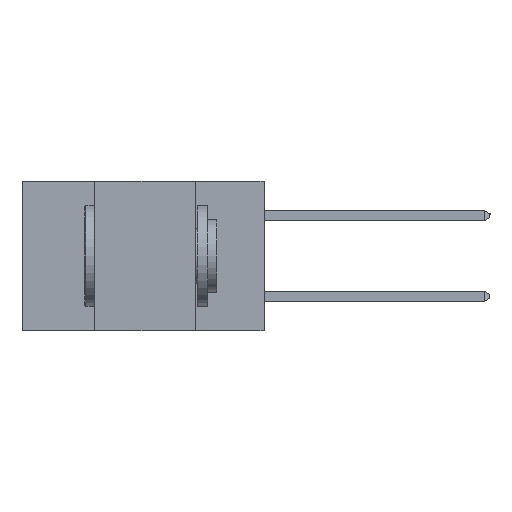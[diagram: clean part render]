
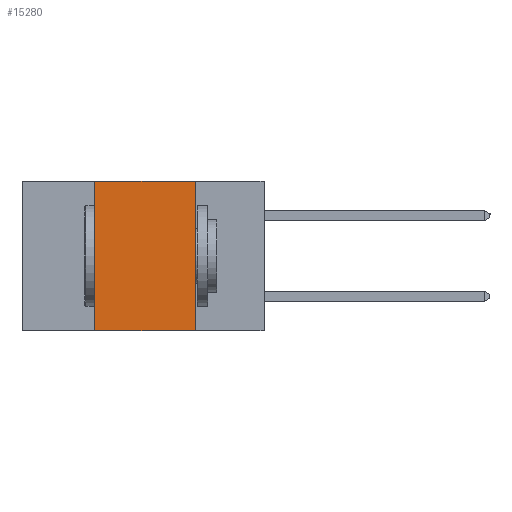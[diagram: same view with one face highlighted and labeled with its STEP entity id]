
A CAD part, left-side view. The second image highlights one B-rep face of the part: STEP entity #15280.
In plain terms, the highlighted planar face has unit normal (-1, 0, 0).
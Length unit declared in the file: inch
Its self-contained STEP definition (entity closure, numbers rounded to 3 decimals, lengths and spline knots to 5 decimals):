
#152 = VECTOR ( 'NONE', #7251, 39.37008 ) ;
#1345 = CARTESIAN_POINT ( 'NONE',  ( 0., 0.17, -0.37 ) ) ;
#1378 = LINE ( 'NONE', #11375, #9827 ) ;
#1451 = DIRECTION ( 'NONE',  ( 0., 0., -1. ) ) ;
#1752 = CARTESIAN_POINT ( 'NONE',  ( 0., 0.17, -0.37 ) ) ;
#1892 = VERTEX_POINT ( 'NONE', #1752 ) ;
#3123 = CARTESIAN_POINT ( 'NONE',  ( 0., 0.42, -0.37 ) ) ;
#3785 = CARTESIAN_POINT ( 'NONE',  ( 0., 0.6, 0. ) ) ;
#4193 = ORIENTED_EDGE ( 'NONE', *, *, #11091, .T. ) ;
#4452 = EDGE_CURVE ( 'NONE', #10727, #8131, #10436, .T. ) ;
#5582 = EDGE_CURVE ( 'NONE', #8131, #6044, #1378, .T. ) ;
#5642 = PLANE ( 'NONE',  #15953 ) ;
#6044 = VERTEX_POINT ( 'NONE', #7387 ) ;
#6091 = CARTESIAN_POINT ( 'NONE',  ( 0., 0.42, -0.37 ) ) ;
#6662 = ORIENTED_EDGE ( 'NONE', *, *, #5582, .F. ) ;
#6948 = DIRECTION ( 'NONE',  ( 0., 0., -1. ) ) ;
#7251 = DIRECTION ( 'NONE',  ( 0., 0., 1. ) ) ;
#7276 = FACE_OUTER_BOUND ( 'NONE', #17084, .T. ) ;
#7387 = CARTESIAN_POINT ( 'NONE',  ( 0., 0.17, 0. ) ) ;
#7412 = LINE ( 'NONE', #1345, #16941 ) ;
#8131 = VERTEX_POINT ( 'NONE', #14866 ) ;
#9384 = DIRECTION ( 'NONE',  ( 0., -1., 0. ) ) ;
#9674 = CARTESIAN_POINT ( 'NONE',  ( 0., 0.6, -0.37 ) ) ;
#9827 = VECTOR ( 'NONE', #9384, 39.37008 ) ;
#10436 = LINE ( 'NONE', #3123, #152 ) ;
#10727 = VERTEX_POINT ( 'NONE', #6091 ) ;
#10775 = ORIENTED_EDGE ( 'NONE', *, *, #13693, .F. ) ;
#11091 = EDGE_CURVE ( 'NONE', #10727, #1892, #13122, .T. ) ;
#11375 = CARTESIAN_POINT ( 'NONE',  ( 0., 0.6, 0. ) ) ;
#12312 = VECTOR ( 'NONE', #16419, 39.37008 ) ;
#13122 = LINE ( 'NONE', #9674, #12312 ) ;
#13693 = EDGE_CURVE ( 'NONE', #6044, #1892, #7412, .T. ) ;
#14866 = CARTESIAN_POINT ( 'NONE',  ( 0., 0.42, 0. ) ) ;
#15280 = ADVANCED_FACE ( 'NONE', ( #7276 ), #5642, .F. ) ;
#15733 = ORIENTED_EDGE ( 'NONE', *, *, #4452, .F. ) ;
#15953 = AXIS2_PLACEMENT_3D ( 'NONE', #3785, #19075, #6948 ) ;
#16419 = DIRECTION ( 'NONE',  ( 0., -1., 0. ) ) ;
#16941 = VECTOR ( 'NONE', #1451, 39.37008 ) ;
#17084 = EDGE_LOOP ( 'NONE', ( #10775, #6662, #15733, #4193 ) ) ;
#19075 = DIRECTION ( 'NONE',  ( 1., 0., 0. ) ) ;
